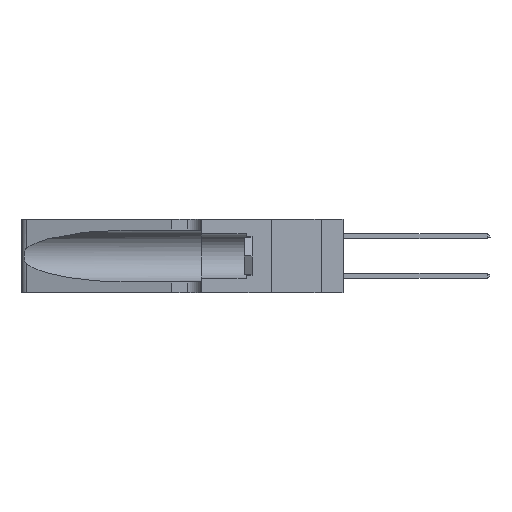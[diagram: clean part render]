
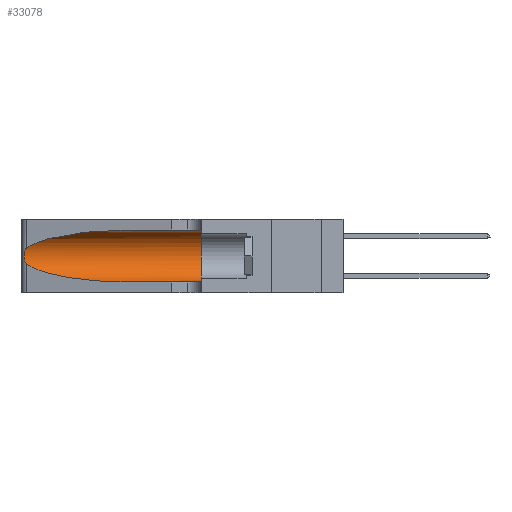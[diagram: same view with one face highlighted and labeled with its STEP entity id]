
A CAD part, left-side view. The second image highlights one B-rep face of the part: STEP entity #33078.
In plain terms, the highlighted cylindrical face has radius 3.308 mm (diameter 6.617 mm), a partial arc.
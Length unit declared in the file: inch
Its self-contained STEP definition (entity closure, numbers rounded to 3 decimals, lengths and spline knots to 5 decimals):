
#1638 = CARTESIAN_POINT ( 'NONE',  ( 0.26075, 1.23896, 0.19203 ) ) ;
#2581 = LINE ( 'NONE', #11109, #37951 ) ;
#3792 = VERTEX_POINT ( 'NONE', #20786 ) ;
#4841 = DIRECTION ( 'NONE',  ( 0., -1., 0. ) ) ;
#5179 = CARTESIAN_POINT ( 'NONE',  ( 0.26017, 1.23833, 0.17102 ) ) ;
#5684 = ORIENTED_EDGE ( 'NONE', *, *, #43281, .T. ) ;
#5714 = AXIS2_PLACEMENT_3D ( 'NONE', #25466, #4841, #28862 ) ;
#8503 = CARTESIAN_POINT ( 'NONE',  ( 0.25555, 1.22994, 0.2215 ) ) ;
#8576 = ORIENTED_EDGE ( 'NONE', *, *, #17706, .F. ) ;
#8648 = CARTESIAN_POINT ( 'NONE',  ( 0.25789, 1.23486, 0.15765 ) ) ;
#8866 = CARTESIAN_POINT ( 'NONE',  ( 0.1305, 0.72297, 0.05475 ) ) ;
#9790 = CARTESIAN_POINT ( 'NONE',  ( 0.25487, 1.22718, 0.14631 ) ) ;
#10127 = DIRECTION ( 'NONE',  ( 0., -1., 0. ) ) ;
#10189 = CARTESIAN_POINT ( 'NONE',  ( 0.25487, 1.22718, 0.22369 ) ) ;
#11109 = CARTESIAN_POINT ( 'NONE',  ( 0.1305, 1.61858, 0.31525 ) ) ;
#11649 = VERTEX_POINT ( 'NONE', #35323 ) ;
#12094 = CARTESIAN_POINT ( 'NONE',  ( 0.25555, 1.22993, 0.14849 ) ) ;
#14524 = LINE ( 'NONE', #27422, #23682 ) ;
#16394 = CARTESIAN_POINT ( 'NONE',  ( 0.1305, 0.72297, 0.31525 ) ) ;
#17706 = EDGE_CURVE ( 'NONE', #11649, #28774, #26453, .T. ) ;
#18211 = DIRECTION ( 'NONE',  ( 0., -1., 0. ) ) ;
#18555 = EDGE_CURVE ( 'NONE', #23367, #43973, #36000, .T. ) ;
#18569 = ORIENTED_EDGE ( 'NONE', *, *, #39955, .T. ) ;
#18847 = CARTESIAN_POINT ( 'NONE',  ( 0.1305, 0.35, 0.185 ) ) ;
#18891 = CARTESIAN_POINT ( 'NONE',  ( 0.25787, 1.23484, 0.2124 ) ) ;
#20438 = CARTESIAN_POINT ( 'NONE',  ( 0.2373, 1.15595, 0.28018 ) ) ;
#20786 = CARTESIAN_POINT ( 'NONE',  ( 0.1305, 0.72297, 0.05475 ) ) ;
#22306 = DIRECTION ( 'NONE',  ( 0., 0., 1. ) ) ;
#22352 = CARTESIAN_POINT ( 'NONE',  ( 0.26018, 1.23835, 0.19895 ) ) ;
#23107 = CYLINDRICAL_SURFACE ( 'NONE', #5714, 0.13025 ) ;
#23367 = VERTEX_POINT ( 'NONE', #16394 ) ;
#23682 = VECTOR ( 'NONE', #10127, 39.37008 ) ;
#24128 = CARTESIAN_POINT ( 'NONE',  ( 0.1305, 0.35, 0.05475 ) ) ;
#24758 = VERTEX_POINT ( 'NONE', #9790 ) ;
#24842 = AXIS2_PLACEMENT_3D ( 'NONE', #18847, #42616, #22306 ) ;
#25251 = FACE_OUTER_BOUND ( 'NONE', #27535, .T. ) ;
#25466 = CARTESIAN_POINT ( 'NONE',  ( 0.1305, 1.61858, 0.185 ) ) ;
#25815 = CARTESIAN_POINT ( 'NONE',  ( 0.26075, 1.23896, 0.178 ) ) ;
#26043 = CARTESIAN_POINT ( 'NONE',  ( 0.25487, 1.22718, 0.14631 ) ) ;
#26453 = CIRCLE ( 'NONE', #24842, 0.13025 ) ;
#26755 = EDGE_CURVE ( 'NONE', #3792, #28774, #14524, .T. ) ;
#27422 = CARTESIAN_POINT ( 'NONE',  ( 0.1305, 1.61858, 0.05475 ) ) ;
#27535 = EDGE_LOOP ( 'NONE', ( #39321, #18569, #5684, #35266, #8576, #40911 ) ) ;
#28774 = VERTEX_POINT ( 'NONE', #24128 ) ;
#28862 = DIRECTION ( 'NONE',  ( 0., 0., -1. ) ) ;
#29194 = CARTESIAN_POINT ( 'NONE',  ( 0.25856, 1.23593, 0.16098 ) ) ;
#29422 = CARTESIAN_POINT ( 'NONE',  ( 0.18966, 0.96281, 0.05475 ) ) ;
#30706 = CARTESIAN_POINT ( 'NONE',  ( 0.1305, 0.72297, 0.31525 ) ) ;
#32598 = CARTESIAN_POINT ( 'NONE',  ( 0.25639, 1.23186, 0.15144 ) ) ;
#33078 = ADVANCED_FACE ( 'NONE', ( #25251 ), #23107, .F. ) ;
#35266 = ORIENTED_EDGE ( 'NONE', *, *, #26755, .T. ) ;
#35323 = CARTESIAN_POINT ( 'NONE',  ( 0.1305, 0.35, 0.31525 ) ) ;
#35837 = CARTESIAN_POINT ( 'NONE',  ( 0.25487, 1.22718, 0.22369 ) ) ;
#35982 = CARTESIAN_POINT ( 'NONE',  ( 0.25487, 1.22718, 0.14631 ) ) ;
#35995 =( BOUNDED_CURVE ( )  B_SPLINE_CURVE ( 3, ( #26043, #42875, #29422, #8866 ),
 .UNSPECIFIED., .F., .F. ) 
 B_SPLINE_CURVE_WITH_KNOTS ( ( 4, 4 ),
 ( 3.44316, 4.71239 ),
 .UNSPECIFIED. ) 
 CURVE ( )  GEOMETRIC_REPRESENTATION_ITEM ( )  RATIONAL_B_SPLINE_CURVE ( ( 1., 0.87, 0.87, 1. ) ) 
 REPRESENTATION_ITEM ( '' )  );
#36000 =( BOUNDED_CURVE ( )  B_SPLINE_CURVE ( 3, ( #30706, #44205, #20438, #10189 ),
 .UNSPECIFIED., .F., .T. ) 
 B_SPLINE_CURVE_WITH_KNOTS ( ( 4, 4 ),
 ( 1.5708, 2.84003 ),
 .UNSPECIFIED. ) 
 CURVE ( )  GEOMETRIC_REPRESENTATION_ITEM ( )  RATIONAL_B_SPLINE_CURVE ( ( 1., 0.87, 0.87, 1. ) ) 
 REPRESENTATION_ITEM ( '' )  );
#37951 = VECTOR ( 'NONE', #18211, 39.37008 ) ;
#39164 = EDGE_CURVE ( 'NONE', #23367, #11649, #2581, .T. ) ;
#39234 = CARTESIAN_POINT ( 'NONE',  ( 0.25639, 1.23184, 0.21858 ) ) ;
#39321 = ORIENTED_EDGE ( 'NONE', *, *, #18555, .T. ) ;
#39955 = EDGE_CURVE ( 'NONE', #43973, #24758, #43336, .T. ) ;
#40911 = ORIENTED_EDGE ( 'NONE', *, *, #39164, .F. ) ;
#42616 = DIRECTION ( 'NONE',  ( 0., 1., 0. ) ) ;
#42659 = CARTESIAN_POINT ( 'NONE',  ( 0.25854, 1.2359, 0.20912 ) ) ;
#42875 = CARTESIAN_POINT ( 'NONE',  ( 0.2373, 1.15595, 0.08982 ) ) ;
#42967 = CARTESIAN_POINT ( 'NONE',  ( 0.25487, 1.22718, 0.22369 ) ) ;
#43281 = EDGE_CURVE ( 'NONE', #24758, #3792, #35995, .T. ) ;
#43336 = B_SPLINE_CURVE_WITH_KNOTS ( 'NONE', 3,
 ( #35837, #8503, #39234, #18891, #42659, #22352, #1638, #25815, #5179, #29194, #8648, #32598, #12094, #35982 ),
 .UNSPECIFIED., .F., .F.,
 ( 4, 2, 2, 2, 2, 2, 4 ),
 ( 0., 0.00027, 0.00053, 0.00107, 0.0016, 0.00187, 0.00214 ),
 .UNSPECIFIED. ) ;
#43973 = VERTEX_POINT ( 'NONE', #42967 ) ;
#44205 = CARTESIAN_POINT ( 'NONE',  ( 0.18966, 0.96281, 0.31525 ) ) ;
